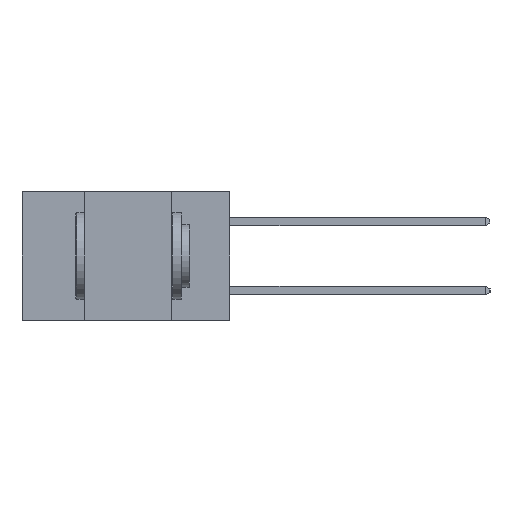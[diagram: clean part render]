
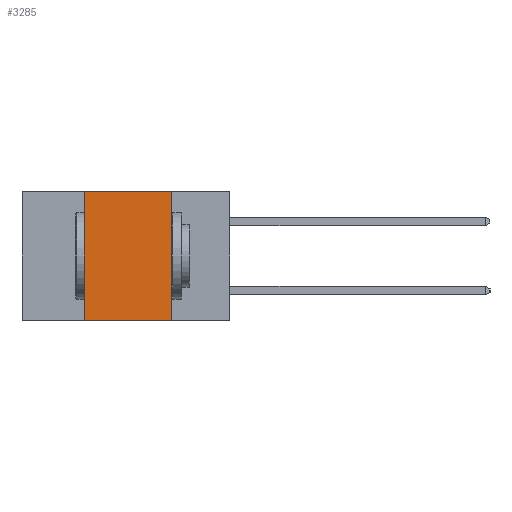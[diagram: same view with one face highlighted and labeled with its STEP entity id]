
A CAD part, left-side view. The second image highlights one B-rep face of the part: STEP entity #3285.
In plain terms, the highlighted planar face has unit normal (-1, 0, 0).
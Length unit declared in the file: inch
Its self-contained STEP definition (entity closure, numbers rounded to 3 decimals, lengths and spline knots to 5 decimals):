
#185 = LINE ( 'NONE', #3016, #664 ) ;
#360 = VECTOR ( 'NONE', #4787, 39.37008 ) ;
#664 = VECTOR ( 'NONE', #13140, 39.37008 ) ;
#1057 = VERTEX_POINT ( 'NONE', #6018 ) ;
#2602 = VECTOR ( 'NONE', #16067, 39.37008 ) ;
#3016 = CARTESIAN_POINT ( 'NONE',  ( 0., 0.42, -0.37 ) ) ;
#3285 = ADVANCED_FACE ( 'NONE', ( #4790 ), #15359, .F. ) ;
#3416 = ORIENTED_EDGE ( 'NONE', *, *, #13001, .F. ) ;
#3644 = VERTEX_POINT ( 'NONE', #8162 ) ;
#4787 = DIRECTION ( 'NONE',  ( 0., -1., 0. ) ) ;
#4790 = FACE_OUTER_BOUND ( 'NONE', #9442, .T. ) ;
#4946 = CARTESIAN_POINT ( 'NONE',  ( 0., 0.6, -0.37 ) ) ;
#5646 = VECTOR ( 'NONE', #6447, 39.37008 ) ;
#5680 = VERTEX_POINT ( 'NONE', #13087 ) ;
#6018 = CARTESIAN_POINT ( 'NONE',  ( 0., 0.42, -0.37 ) ) ;
#6447 = DIRECTION ( 'NONE',  ( 0., -1., 0. ) ) ;
#6911 = ORIENTED_EDGE ( 'NONE', *, *, #8622, .F. ) ;
#8162 = CARTESIAN_POINT ( 'NONE',  ( 0., 0.17, -0.37 ) ) ;
#8230 = LINE ( 'NONE', #13395, #360 ) ;
#8622 = EDGE_CURVE ( 'NONE', #1057, #5680, #185, .T. ) ;
#9442 = EDGE_LOOP ( 'NONE', ( #14903, #3416, #6911, #17564 ) ) ;
#9553 = LINE ( 'NONE', #4946, #5646 ) ;
#10110 = CARTESIAN_POINT ( 'NONE',  ( 0., 0.17, 0. ) ) ;
#13001 = EDGE_CURVE ( 'NONE', #5680, #13982, #8230, .T. ) ;
#13087 = CARTESIAN_POINT ( 'NONE',  ( 0., 0.42, 0. ) ) ;
#13140 = DIRECTION ( 'NONE',  ( 0., 0., 1. ) ) ;
#13395 = CARTESIAN_POINT ( 'NONE',  ( 0., 0.6, 0. ) ) ;
#13982 = VERTEX_POINT ( 'NONE', #10110 ) ;
#14191 = EDGE_CURVE ( 'NONE', #13982, #3644, #17274, .T. ) ;
#14300 = DIRECTION ( 'NONE',  ( 0., 0., -1. ) ) ;
#14315 = DIRECTION ( 'NONE',  ( 1., 0., 0. ) ) ;
#14423 = CARTESIAN_POINT ( 'NONE',  ( 0., 0.6, 0. ) ) ;
#14715 = CARTESIAN_POINT ( 'NONE',  ( 0., 0.17, -0.37 ) ) ;
#14903 = ORIENTED_EDGE ( 'NONE', *, *, #14191, .F. ) ;
#15359 = PLANE ( 'NONE',  #16890 ) ;
#16067 = DIRECTION ( 'NONE',  ( 0., 0., -1. ) ) ;
#16890 = AXIS2_PLACEMENT_3D ( 'NONE', #14423, #14315, #14300 ) ;
#17274 = LINE ( 'NONE', #14715, #2602 ) ;
#17532 = EDGE_CURVE ( 'NONE', #1057, #3644, #9553, .T. ) ;
#17564 = ORIENTED_EDGE ( 'NONE', *, *, #17532, .T. ) ;
